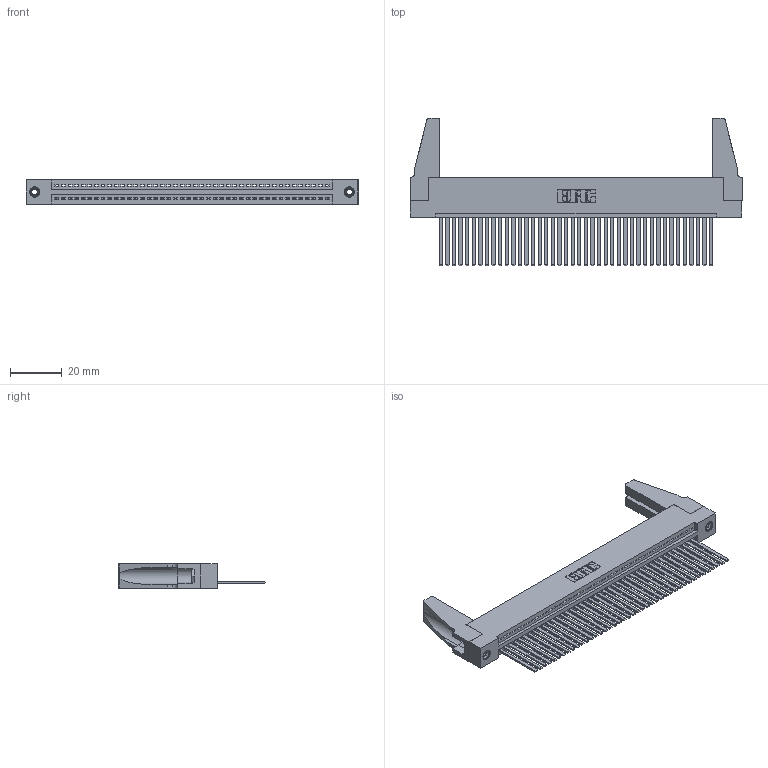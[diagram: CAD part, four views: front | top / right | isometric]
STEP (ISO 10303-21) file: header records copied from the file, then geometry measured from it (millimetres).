
FILE_DESCRIPTION (( 'STEP AP203' ), '1' );
FILE_NAME ('345-042-544-188.STEP', '2019-10-08T15:08:20', ( '' ), ( '' ), 'SwSTEP 2.0', 'SolidWorks 2016', '' );
FILE_SCHEMA (( 'CONFIG_CONTROL_DESIGN' ));
Length unit declared in the file: inch
Products named in the file (5): 345-042-544-188; 345-292-001_345-293-144; 345 Part_Flush Mounting Lugs - 0.156 Dia-TH; 345-220-078_345-220-088; 345-250-001_345-250-001-102
Assembly tree (47 placements, depth 2):
  345-042-544-188
    345 Part_Flush Mounting Lugs - 0.156 Dia-TH
    345-292-001_345-293-144  x42
    345-250-001_345-250-001-102  x2
    345-220-078_345-220-088  x2
Bounding box: 127.91 x 56.82 x 9.4 mm (x, y, z)
Volume: 15888.4 mm3; surface area: 21381.4 mm2
Topology: 47 solids, 47 shells, 2434 faces, 7291 edges, 4794 vertices
Faces by surface type: plane 1664, cylinder 754, cone 12, torus 4
Entity records: 33574 total; most frequent: CARTESIAN_POINT 5804, ORIENTED_EDGE 5740, DIRECTION 5074, EDGE_CURVE 2870, LINE 2532, VECTOR 2532, VERTEX_POINT 1906, AXIS2_PLACEMENT_3D 1271
